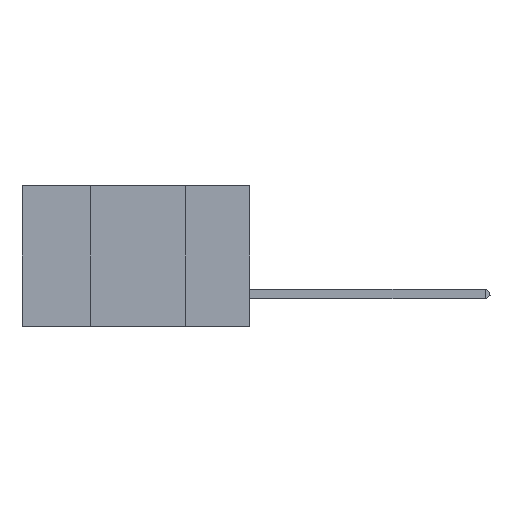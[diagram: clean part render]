
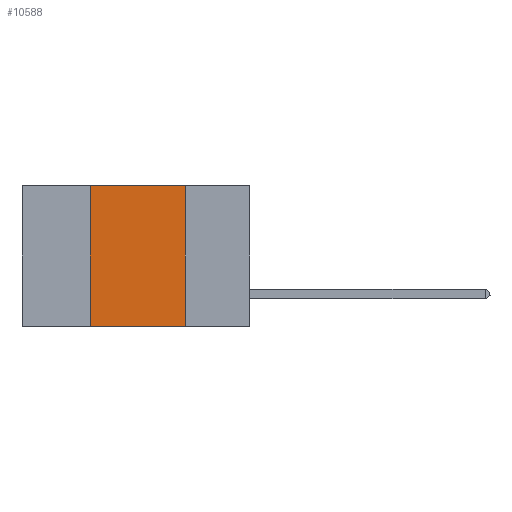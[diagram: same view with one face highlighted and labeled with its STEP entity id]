
A CAD part, left-side view. The second image highlights one B-rep face of the part: STEP entity #10588.
In plain terms, the highlighted planar face has unit normal (-1, 0, 0).
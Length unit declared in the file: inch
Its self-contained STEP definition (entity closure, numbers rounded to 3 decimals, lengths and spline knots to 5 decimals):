
#10 = DIRECTION ( 'NONE',  ( 0., -1., 0. ) ) ;
#1017 = EDGE_CURVE ( 'NONE', #10263, #17834, #20127, .T. ) ;
#2256 = ORIENTED_EDGE ( 'NONE', *, *, #15226, .F. ) ;
#2940 = EDGE_CURVE ( 'NONE', #23667, #28402, #20400, .T. ) ;
#4809 = ORIENTED_EDGE ( 'NONE', *, *, #1017, .F. ) ;
#5544 = VECTOR ( 'NONE', #19564, 39.37008 ) ;
#5768 = DIRECTION ( 'NONE',  ( 0., 0., -1. ) ) ;
#6256 = EDGE_LOOP ( 'NONE', ( #11746, #4809, #2256, #14245 ) ) ;
#7635 = PLANE ( 'NONE',  #13261 ) ;
#7652 = LINE ( 'NONE', #21837, #5544 ) ;
#9227 = CARTESIAN_POINT ( 'NONE',  ( 0., 0.42, -0.37 ) ) ;
#9776 = EDGE_CURVE ( 'NONE', #17834, #28402, #14865, .T. ) ;
#10263 = VERTEX_POINT ( 'NONE', #13598 ) ;
#10588 = ADVANCED_FACE ( 'NONE', ( #27967 ), #7635, .F. ) ;
#11537 = CARTESIAN_POINT ( 'NONE',  ( 0., 0.6, 0. ) ) ;
#11746 = ORIENTED_EDGE ( 'NONE', *, *, #9776, .F. ) ;
#13261 = AXIS2_PLACEMENT_3D ( 'NONE', #25617, #23089, #16635 ) ;
#13598 = CARTESIAN_POINT ( 'NONE',  ( 0., 0.42, 0. ) ) ;
#14245 = ORIENTED_EDGE ( 'NONE', *, *, #2940, .T. ) ;
#14865 = LINE ( 'NONE', #16733, #18330 ) ;
#14981 = CARTESIAN_POINT ( 'NONE',  ( 0., 0.17, 0. ) ) ;
#15210 = CARTESIAN_POINT ( 'NONE',  ( 0., 0.6, -0.37 ) ) ;
#15226 = EDGE_CURVE ( 'NONE', #23667, #10263, #7652, .T. ) ;
#16635 = DIRECTION ( 'NONE',  ( 0., 0., -1. ) ) ;
#16733 = CARTESIAN_POINT ( 'NONE',  ( 0., 0.17, 0. ) ) ;
#17834 = VERTEX_POINT ( 'NONE', #14981 ) ;
#18330 = VECTOR ( 'NONE', #5768, 39.37008 ) ;
#19564 = DIRECTION ( 'NONE',  ( 0., 0., 1. ) ) ;
#20127 = LINE ( 'NONE', #11537, #27050 ) ;
#20400 = LINE ( 'NONE', #15210, #22481 ) ;
#20703 = DIRECTION ( 'NONE',  ( 0., -1., 0. ) ) ;
#21837 = CARTESIAN_POINT ( 'NONE',  ( 0., 0.42, 0. ) ) ;
#22481 = VECTOR ( 'NONE', #10, 39.37008 ) ;
#23089 = DIRECTION ( 'NONE',  ( 1., 0., 0. ) ) ;
#23667 = VERTEX_POINT ( 'NONE', #9227 ) ;
#25078 = CARTESIAN_POINT ( 'NONE',  ( 0., 0.17, -0.37 ) ) ;
#25617 = CARTESIAN_POINT ( 'NONE',  ( 0., 0.6, 0. ) ) ;
#27050 = VECTOR ( 'NONE', #20703, 39.37008 ) ;
#27967 = FACE_OUTER_BOUND ( 'NONE', #6256, .T. ) ;
#28402 = VERTEX_POINT ( 'NONE', #25078 ) ;
